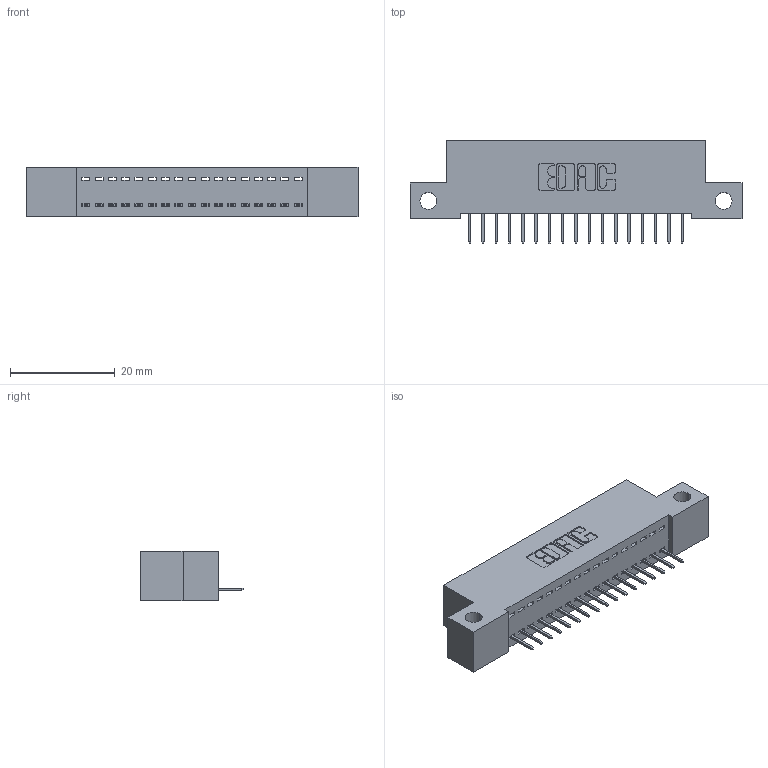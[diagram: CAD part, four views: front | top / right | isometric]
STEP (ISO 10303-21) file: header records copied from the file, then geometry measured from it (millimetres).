
FILE_DESCRIPTION (( 'STEP AP203' ), '1' );
FILE_NAME ('342-017-524-112.STEP', '2019-10-01T19:25:23', ( '' ), ( '' ), 'SwSTEP 2.0', 'SolidWorks 2016', '' );
FILE_SCHEMA (( 'CONFIG_CONTROL_DESIGN' ));
Length unit declared in the file: inch
Products named in the file (3): 345-292-001_345-293-124; 342-017-524-112; 342 Part_Side Mount
Assembly tree (18 placements, depth 2):
  342-017-524-112
    342 Part_Side Mount
    345-292-001_345-293-124  x17
Bounding box: 63.5 x 19.69 x 9.4 mm (x, y, z)
Volume: 5334.5 mm3; surface area: 6995 mm2
Topology: 18 solids, 18 shells, 1164 faces, 3359 edges, 2170 vertices
Faces by surface type: plane 882, cylinder 282
Entity records: 13571 total; most frequent: CARTESIAN_POINT 2349, ORIENTED_EDGE 2302, DIRECTION 2033, EDGE_CURVE 1151, VECTOR 1027, LINE 1027, VERTEX_POINT 762, AXIS2_PLACEMENT_3D 503
